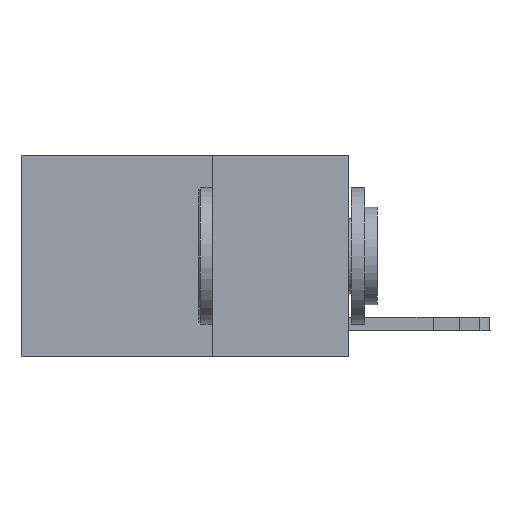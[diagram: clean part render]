
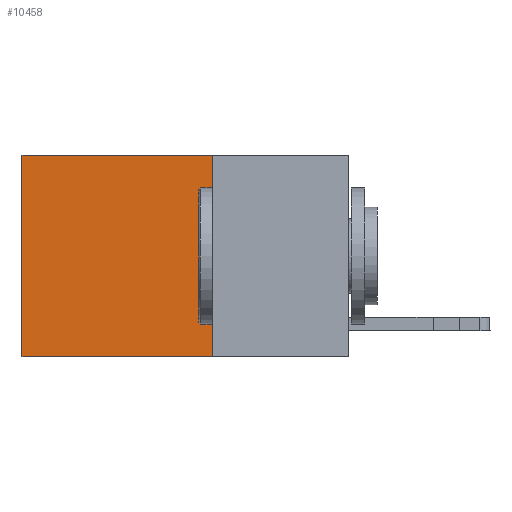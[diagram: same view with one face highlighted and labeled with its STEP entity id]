
A CAD part, left-side view. The second image highlights one B-rep face of the part: STEP entity #10458.
In plain terms, the highlighted planar face has unit normal (-1, 0, 0).
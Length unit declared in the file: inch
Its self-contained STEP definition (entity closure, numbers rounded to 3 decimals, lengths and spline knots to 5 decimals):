
#132 = ORIENTED_EDGE ( 'NONE', *, *, #3628, .F. ) ;
#760 = CARTESIAN_POINT ( 'NONE',  ( 0.2625, 0.6, 0. ) ) ;
#872 = VERTEX_POINT ( 'NONE', #997 ) ;
#900 = LINE ( 'NONE', #7219, #3591 ) ;
#997 = CARTESIAN_POINT ( 'NONE',  ( 0.2625, 0.25, -0.37 ) ) ;
#1263 = VECTOR ( 'NONE', #12288, 39.37008 ) ;
#1538 = DIRECTION ( 'NONE',  ( 1., 0., 0. ) ) ;
#1594 = CARTESIAN_POINT ( 'NONE',  ( 0.2625, 0.25, 0. ) ) ;
#2428 = LINE ( 'NONE', #7432, #5154 ) ;
#2802 = EDGE_CURVE ( 'NONE', #10562, #4998, #900, .T. ) ;
#2874 = CARTESIAN_POINT ( 'NONE',  ( 0.2625, 0.25, 0. ) ) ;
#2928 = DIRECTION ( 'NONE',  ( 0., 0., -1. ) ) ;
#3535 = CARTESIAN_POINT ( 'NONE',  ( 0.2625, 0.25, 0. ) ) ;
#3591 = VECTOR ( 'NONE', #7605, 39.37008 ) ;
#3628 = EDGE_CURVE ( 'NONE', #872, #4998, #2428, .T. ) ;
#4140 = AXIS2_PLACEMENT_3D ( 'NONE', #3535, #1538, #8427 ) ;
#4178 = EDGE_LOOP ( 'NONE', ( #11367, #132, #7124, #4265 ) ) ;
#4265 = ORIENTED_EDGE ( 'NONE', *, *, #5710, .T. ) ;
#4632 = FACE_OUTER_BOUND ( 'NONE', #4178, .T. ) ;
#4644 = LINE ( 'NONE', #2874, #9417 ) ;
#4815 = CARTESIAN_POINT ( 'NONE',  ( 0.2625, 0.6, -0.37 ) ) ;
#4998 = VERTEX_POINT ( 'NONE', #4815 ) ;
#5154 = VECTOR ( 'NONE', #7629, 39.37008 ) ;
#5635 = VERTEX_POINT ( 'NONE', #12169 ) ;
#5710 = EDGE_CURVE ( 'NONE', #5635, #10562, #8206, .T. ) ;
#7124 = ORIENTED_EDGE ( 'NONE', *, *, #10030, .F. ) ;
#7219 = CARTESIAN_POINT ( 'NONE',  ( 0.2625, 0.6, 0. ) ) ;
#7432 = CARTESIAN_POINT ( 'NONE',  ( 0.2625, 0.25, -0.37 ) ) ;
#7471 = PLANE ( 'NONE',  #4140 ) ;
#7605 = DIRECTION ( 'NONE',  ( 0., 0., -1. ) ) ;
#7629 = DIRECTION ( 'NONE',  ( 0., 1., 0. ) ) ;
#8206 = LINE ( 'NONE', #1594, #1263 ) ;
#8427 = DIRECTION ( 'NONE',  ( 0., 0., -1. ) ) ;
#9417 = VECTOR ( 'NONE', #2928, 39.37008 ) ;
#10030 = EDGE_CURVE ( 'NONE', #5635, #872, #4644, .T. ) ;
#10458 = ADVANCED_FACE ( 'NONE', ( #4632 ), #7471, .F. ) ;
#10562 = VERTEX_POINT ( 'NONE', #760 ) ;
#11367 = ORIENTED_EDGE ( 'NONE', *, *, #2802, .T. ) ;
#12169 = CARTESIAN_POINT ( 'NONE',  ( 0.2625, 0.25, 0. ) ) ;
#12288 = DIRECTION ( 'NONE',  ( 0., 1., 0. ) ) ;
